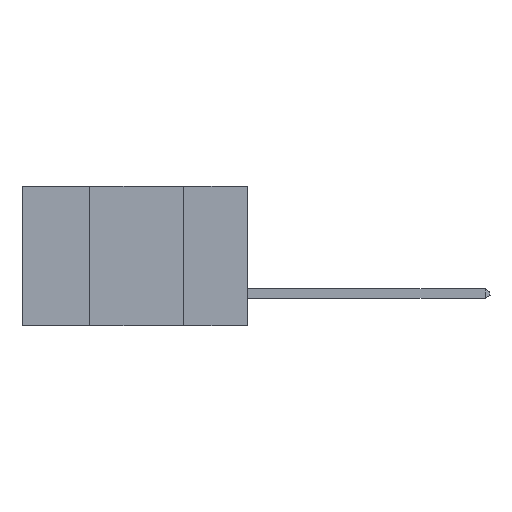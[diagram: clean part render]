
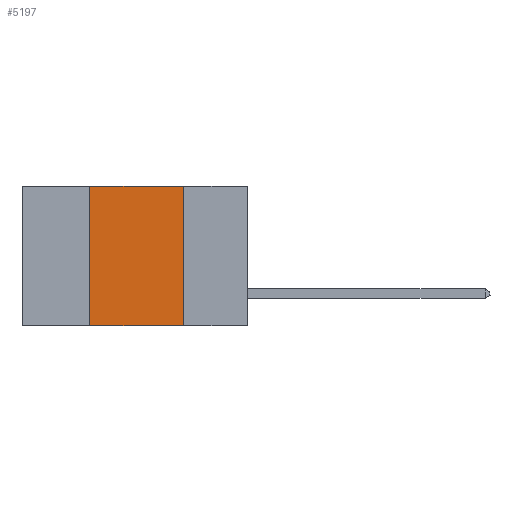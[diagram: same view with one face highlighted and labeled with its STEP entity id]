
A CAD part, left-side view. The second image highlights one B-rep face of the part: STEP entity #5197.
In plain terms, the highlighted planar face has unit normal (-1, 0, 0).
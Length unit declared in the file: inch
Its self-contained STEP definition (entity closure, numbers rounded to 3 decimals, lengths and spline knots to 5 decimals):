
#45 = EDGE_CURVE ( 'NONE', #5391, #11661, #7652, .T. ) ;
#82 = CARTESIAN_POINT ( 'NONE',  ( 0., 0.17, -0.37 ) ) ;
#578 = CARTESIAN_POINT ( 'NONE',  ( 0., 0.42, 0. ) ) ;
#1240 = VERTEX_POINT ( 'NONE', #10154 ) ;
#2025 = VECTOR ( 'NONE', #2396, 39.37008 ) ;
#2153 = VECTOR ( 'NONE', #9416, 39.37008 ) ;
#2396 = DIRECTION ( 'NONE',  ( 0., -1., 0. ) ) ;
#2451 = EDGE_CURVE ( 'NONE', #1240, #10495, #5036, .T. ) ;
#2516 = DIRECTION ( 'NONE',  ( 1., 0., 0. ) ) ;
#2523 = ORIENTED_EDGE ( 'NONE', *, *, #10257, .F. ) ;
#2774 = CARTESIAN_POINT ( 'NONE',  ( 0., 0.6, 0. ) ) ;
#3266 = EDGE_CURVE ( 'NONE', #5391, #1240, #4732, .T. ) ;
#4732 = LINE ( 'NONE', #578, #2153 ) ;
#5036 = LINE ( 'NONE', #2774, #8949 ) ;
#5057 = CARTESIAN_POINT ( 'NONE',  ( 0., 0.42, -0.37 ) ) ;
#5197 = ADVANCED_FACE ( 'NONE', ( #14064 ), #8046, .F. ) ;
#5391 = VERTEX_POINT ( 'NONE', #5057 ) ;
#6305 = ORIENTED_EDGE ( 'NONE', *, *, #45, .T. ) ;
#6352 = DIRECTION ( 'NONE',  ( 0., 0., -1. ) ) ;
#6849 = EDGE_LOOP ( 'NONE', ( #2523, #13616, #12257, #6305 ) ) ;
#6885 = CARTESIAN_POINT ( 'NONE',  ( 0., 0.6, 0. ) ) ;
#7147 = AXIS2_PLACEMENT_3D ( 'NONE', #6885, #2516, #11260 ) ;
#7652 = LINE ( 'NONE', #10247, #2025 ) ;
#8046 = PLANE ( 'NONE',  #7147 ) ;
#8857 = VECTOR ( 'NONE', #6352, 39.37008 ) ;
#8949 = VECTOR ( 'NONE', #9276, 39.37008 ) ;
#9276 = DIRECTION ( 'NONE',  ( 0., -1., 0. ) ) ;
#9416 = DIRECTION ( 'NONE',  ( 0., 0., 1. ) ) ;
#9552 = CARTESIAN_POINT ( 'NONE',  ( 0., 0.17, 0. ) ) ;
#10070 = LINE ( 'NONE', #13978, #8857 ) ;
#10154 = CARTESIAN_POINT ( 'NONE',  ( 0., 0.42, 0. ) ) ;
#10247 = CARTESIAN_POINT ( 'NONE',  ( 0., 0.6, -0.37 ) ) ;
#10257 = EDGE_CURVE ( 'NONE', #10495, #11661, #10070, .T. ) ;
#10495 = VERTEX_POINT ( 'NONE', #9552 ) ;
#11260 = DIRECTION ( 'NONE',  ( 0., 0., -1. ) ) ;
#11661 = VERTEX_POINT ( 'NONE', #82 ) ;
#12257 = ORIENTED_EDGE ( 'NONE', *, *, #3266, .F. ) ;
#13616 = ORIENTED_EDGE ( 'NONE', *, *, #2451, .F. ) ;
#13978 = CARTESIAN_POINT ( 'NONE',  ( 0., 0.17, 0. ) ) ;
#14064 = FACE_OUTER_BOUND ( 'NONE', #6849, .T. ) ;
